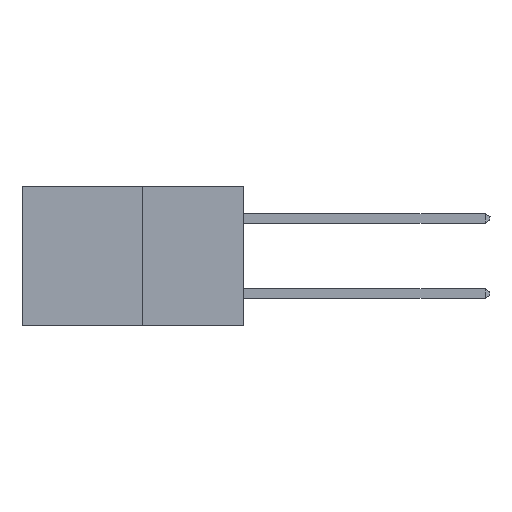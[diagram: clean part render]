
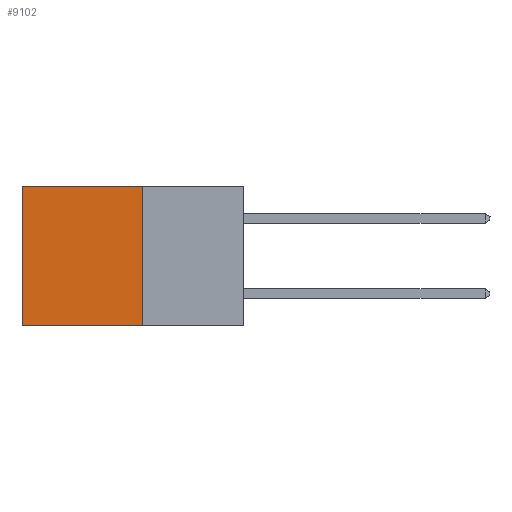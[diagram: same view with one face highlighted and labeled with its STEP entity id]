
A CAD part, left-side view. The second image highlights one B-rep face of the part: STEP entity #9102.
In plain terms, the highlighted planar face has unit normal (-1, 0, 0).
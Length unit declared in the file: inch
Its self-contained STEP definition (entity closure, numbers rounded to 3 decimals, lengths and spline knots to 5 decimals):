
#292 = EDGE_CURVE ( 'NONE', #5989, #5766, #31679, .T. ) ;
#472 = LINE ( 'NONE', #20815, #28723 ) ;
#820 = LINE ( 'NONE', #1636, #28209 ) ;
#1044 = CARTESIAN_POINT ( 'NONE',  ( 0.277, 0.59, 0. ) ) ;
#1433 = DIRECTION ( 'NONE',  ( 0., 0., -1. ) ) ;
#1636 = CARTESIAN_POINT ( 'NONE',  ( 0.277, 0.27, -0.37 ) ) ;
#3132 = CARTESIAN_POINT ( 'NONE',  ( 0.277, 0.59, -0.37 ) ) ;
#3567 = VERTEX_POINT ( 'NONE', #24970 ) ;
#3803 = EDGE_CURVE ( 'NONE', #3567, #5766, #472, .T. ) ;
#4959 = EDGE_CURVE ( 'NONE', #31362, #3567, #820, .T. ) ;
#4990 = DIRECTION ( 'NONE',  ( 0., 0., -1. ) ) ;
#5766 = VERTEX_POINT ( 'NONE', #3132 ) ;
#5989 = VERTEX_POINT ( 'NONE', #1044 ) ;
#7293 = ORIENTED_EDGE ( 'NONE', *, *, #4959, .F. ) ;
#7471 = CARTESIAN_POINT ( 'NONE',  ( 0.277, 0.59, -0.37 ) ) ;
#7502 = EDGE_CURVE ( 'NONE', #31362, #5989, #25504, .T. ) ;
#7520 = DIRECTION ( 'NONE',  ( 0., 0., -1. ) ) ;
#9102 = ADVANCED_FACE ( 'NONE', ( #18565 ), #32114, .F. ) ;
#10359 = ORIENTED_EDGE ( 'NONE', *, *, #3803, .F. ) ;
#12449 = CARTESIAN_POINT ( 'NONE',  ( 0.277, 0.27, 0. ) ) ;
#13957 = AXIS2_PLACEMENT_3D ( 'NONE', #29391, #21295, #4990 ) ;
#16336 = VECTOR ( 'NONE', #7520, 39.37008 ) ;
#18255 = VECTOR ( 'NONE', #23471, 39.37008 ) ;
#18565 = FACE_OUTER_BOUND ( 'NONE', #27518, .T. ) ;
#18971 = ORIENTED_EDGE ( 'NONE', *, *, #292, .T. ) ;
#20587 = DIRECTION ( 'NONE',  ( 0., 1., 0. ) ) ;
#20815 = CARTESIAN_POINT ( 'NONE',  ( 0.277, 0.27, -0.37 ) ) ;
#21295 = DIRECTION ( 'NONE',  ( 1., 0., 0. ) ) ;
#23471 = DIRECTION ( 'NONE',  ( 0., 1., 0. ) ) ;
#24970 = CARTESIAN_POINT ( 'NONE',  ( 0.277, 0.27, -0.37 ) ) ;
#25504 = LINE ( 'NONE', #12449, #18255 ) ;
#27518 = EDGE_LOOP ( 'NONE', ( #18971, #10359, #7293, #30286 ) ) ;
#28209 = VECTOR ( 'NONE', #1433, 39.37008 ) ;
#28723 = VECTOR ( 'NONE', #20587, 39.37008 ) ;
#29391 = CARTESIAN_POINT ( 'NONE',  ( 0.277, 0.27, -0.37 ) ) ;
#30286 = ORIENTED_EDGE ( 'NONE', *, *, #7502, .T. ) ;
#31362 = VERTEX_POINT ( 'NONE', #35270 ) ;
#31679 = LINE ( 'NONE', #7471, #16336 ) ;
#32114 = PLANE ( 'NONE',  #13957 ) ;
#35270 = CARTESIAN_POINT ( 'NONE',  ( 0.277, 0.27, 0. ) ) ;
